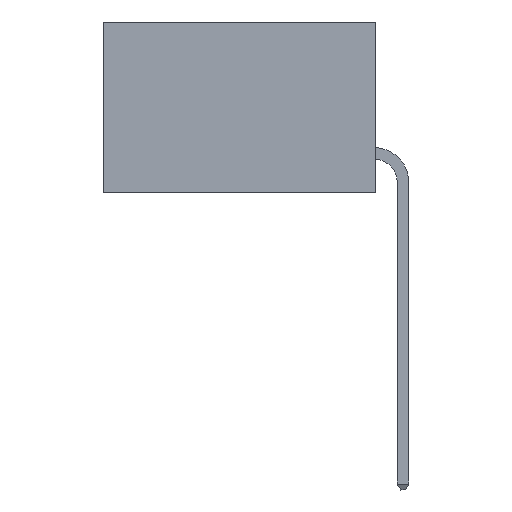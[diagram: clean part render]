
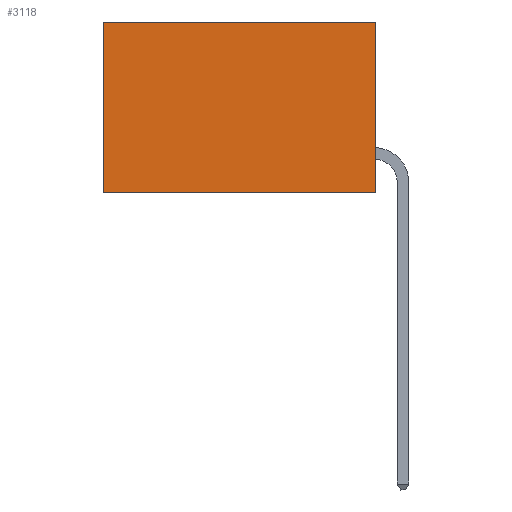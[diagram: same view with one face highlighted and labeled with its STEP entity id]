
A CAD part, left-side view. The second image highlights one B-rep face of the part: STEP entity #3118.
In plain terms, the highlighted planar face has unit normal (-1, 0, 0).
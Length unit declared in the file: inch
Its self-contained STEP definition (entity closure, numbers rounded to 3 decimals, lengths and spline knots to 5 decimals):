
#503 = PLANE ( 'NONE',  #7640 ) ;
#789 = CARTESIAN_POINT ( 'NONE',  ( 0.277, 0.59, -0.37 ) ) ;
#1152 = CARTESIAN_POINT ( 'NONE',  ( 0.277, 0., -0.37 ) ) ;
#1199 = VERTEX_POINT ( 'NONE', #6885 ) ;
#1214 = ORIENTED_EDGE ( 'NONE', *, *, #7163, .F. ) ;
#1426 = CARTESIAN_POINT ( 'NONE',  ( 0.277, 0., -0.37 ) ) ;
#1443 = VECTOR ( 'NONE', #5786, 39.37008 ) ;
#1627 = VERTEX_POINT ( 'NONE', #789 ) ;
#1775 = ORIENTED_EDGE ( 'NONE', *, *, #9178, .F. ) ;
#1794 = DIRECTION ( 'NONE',  ( 0., 0., -1. ) ) ;
#2037 = CARTESIAN_POINT ( 'NONE',  ( 0.277, 0., -0.37 ) ) ;
#2114 = DIRECTION ( 'NONE',  ( 0., 0., -1. ) ) ;
#2391 = VECTOR ( 'NONE', #6940, 39.37008 ) ;
#2645 = ORIENTED_EDGE ( 'NONE', *, *, #3081, .T. ) ;
#2999 = DIRECTION ( 'NONE',  ( 1., 0., 0. ) ) ;
#3007 = LINE ( 'NONE', #4060, #4713 ) ;
#3081 = EDGE_CURVE ( 'NONE', #1199, #1627, #6756, .T. ) ;
#3118 = ADVANCED_FACE ( 'NONE', ( #4725 ), #503, .F. ) ;
#4060 = CARTESIAN_POINT ( 'NONE',  ( 0.277, 0., 0. ) ) ;
#4074 = DIRECTION ( 'NONE',  ( 0., 1., 0. ) ) ;
#4342 = LINE ( 'NONE', #1152, #2391 ) ;
#4564 = ORIENTED_EDGE ( 'NONE', *, *, #7237, .T. ) ;
#4713 = VECTOR ( 'NONE', #4074, 39.37008 ) ;
#4725 = FACE_OUTER_BOUND ( 'NONE', #8341, .T. ) ;
#5216 = CARTESIAN_POINT ( 'NONE',  ( 0.277, 0.59, -0.37 ) ) ;
#5786 = DIRECTION ( 'NONE',  ( 0., 0., -1. ) ) ;
#5857 = CARTESIAN_POINT ( 'NONE',  ( 0.277, 0., -0.37 ) ) ;
#6756 = LINE ( 'NONE', #5216, #7176 ) ;
#6885 = CARTESIAN_POINT ( 'NONE',  ( 0.277, 0.59, 0. ) ) ;
#6940 = DIRECTION ( 'NONE',  ( 0., 1., 0. ) ) ;
#7163 = EDGE_CURVE ( 'NONE', #9261, #8293, #8879, .T. ) ;
#7176 = VECTOR ( 'NONE', #1794, 39.37008 ) ;
#7237 = EDGE_CURVE ( 'NONE', #9261, #1199, #3007, .T. ) ;
#7640 = AXIS2_PLACEMENT_3D ( 'NONE', #1426, #2999, #2114 ) ;
#8293 = VERTEX_POINT ( 'NONE', #2037 ) ;
#8341 = EDGE_LOOP ( 'NONE', ( #2645, #1775, #1214, #4564 ) ) ;
#8879 = LINE ( 'NONE', #5857, #1443 ) ;
#8942 = CARTESIAN_POINT ( 'NONE',  ( 0.277, 0., 0. ) ) ;
#9178 = EDGE_CURVE ( 'NONE', #8293, #1627, #4342, .T. ) ;
#9261 = VERTEX_POINT ( 'NONE', #8942 ) ;
